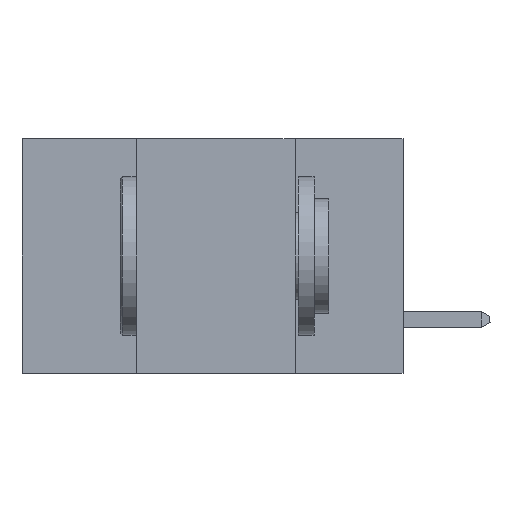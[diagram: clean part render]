
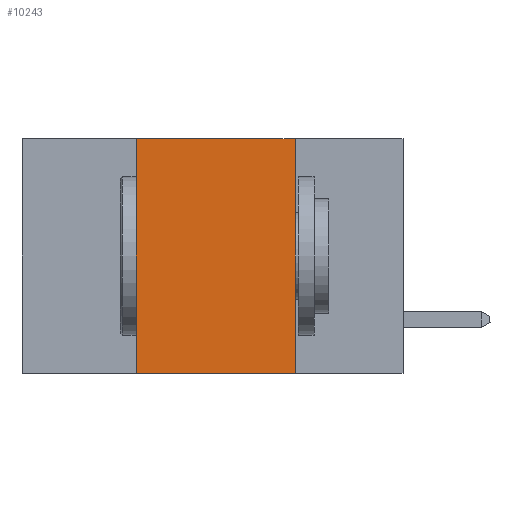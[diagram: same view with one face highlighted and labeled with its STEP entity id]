
A CAD part, left-side view. The second image highlights one B-rep face of the part: STEP entity #10243.
In plain terms, the highlighted planar face has unit normal (-1, 0, 0).
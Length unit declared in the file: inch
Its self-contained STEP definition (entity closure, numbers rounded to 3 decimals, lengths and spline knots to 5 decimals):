
#79 = CARTESIAN_POINT ( 'NONE',  ( 0., 0.6, 0. ) ) ;
#417 = CARTESIAN_POINT ( 'NONE',  ( 0., 0.6, -0.37 ) ) ;
#625 = CARTESIAN_POINT ( 'NONE',  ( 0., 0.42, -0.37 ) ) ;
#1135 = DIRECTION ( 'NONE',  ( 0., -1., 0. ) ) ;
#2107 = DIRECTION ( 'NONE',  ( 0., 0., -1. ) ) ;
#2857 = CARTESIAN_POINT ( 'NONE',  ( 0., 0.17, 0. ) ) ;
#3178 = CARTESIAN_POINT ( 'NONE',  ( 0., 0.6, 0. ) ) ;
#3956 = VECTOR ( 'NONE', #1135, 39.37008 ) ;
#4973 = FACE_OUTER_BOUND ( 'NONE', #7174, .T. ) ;
#5068 = DIRECTION ( 'NONE',  ( 0., -1., 0. ) ) ;
#5544 = CARTESIAN_POINT ( 'NONE',  ( 0., 0.17, -0.37 ) ) ;
#5744 = VERTEX_POINT ( 'NONE', #2857 ) ;
#6496 = LINE ( 'NONE', #12234, #11129 ) ;
#6497 = DIRECTION ( 'NONE',  ( 1., 0., 0. ) ) ;
#7174 = EDGE_LOOP ( 'NONE', ( #14289, #12577, #11614, #11428 ) ) ;
#7839 = LINE ( 'NONE', #16695, #20172 ) ;
#8526 = EDGE_CURVE ( 'NONE', #17082, #5744, #19371, .T. ) ;
#9393 = DIRECTION ( 'NONE',  ( 0., 0., 1. ) ) ;
#10243 = ADVANCED_FACE ( 'NONE', ( #4973 ), #17609, .F. ) ;
#10373 = CARTESIAN_POINT ( 'NONE',  ( 0., 0.42, 0. ) ) ;
#11129 = VECTOR ( 'NONE', #9393, 39.37008 ) ;
#11428 = ORIENTED_EDGE ( 'NONE', *, *, #13728, .T. ) ;
#11614 = ORIENTED_EDGE ( 'NONE', *, *, #13489, .F. ) ;
#12234 = CARTESIAN_POINT ( 'NONE',  ( 0., 0.42, 0. ) ) ;
#12475 = EDGE_CURVE ( 'NONE', #5744, #15112, #7839, .T. ) ;
#12577 = ORIENTED_EDGE ( 'NONE', *, *, #8526, .F. ) ;
#12627 = LINE ( 'NONE', #417, #3956 ) ;
#12690 = VECTOR ( 'NONE', #5068, 39.37008 ) ;
#13489 = EDGE_CURVE ( 'NONE', #15336, #17082, #6496, .T. ) ;
#13728 = EDGE_CURVE ( 'NONE', #15336, #15112, #12627, .T. ) ;
#14289 = ORIENTED_EDGE ( 'NONE', *, *, #12475, .F. ) ;
#15112 = VERTEX_POINT ( 'NONE', #5544 ) ;
#15336 = VERTEX_POINT ( 'NONE', #625 ) ;
#16695 = CARTESIAN_POINT ( 'NONE',  ( 0., 0.17, 0. ) ) ;
#17082 = VERTEX_POINT ( 'NONE', #10373 ) ;
#17609 = PLANE ( 'NONE',  #18548 ) ;
#17956 = DIRECTION ( 'NONE',  ( 0., 0., -1. ) ) ;
#18548 = AXIS2_PLACEMENT_3D ( 'NONE', #3178, #6497, #17956 ) ;
#19371 = LINE ( 'NONE', #79, #12690 ) ;
#20172 = VECTOR ( 'NONE', #2107, 39.37008 ) ;
